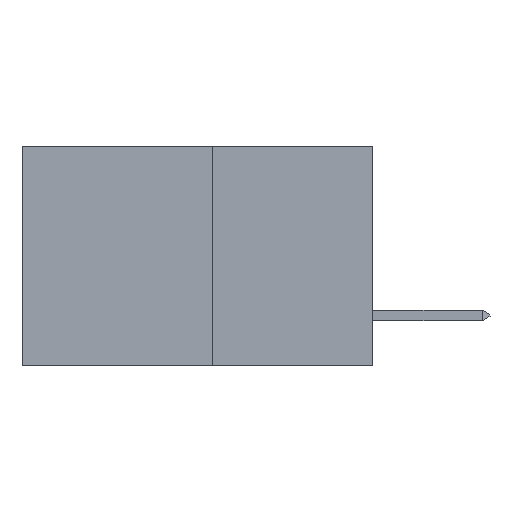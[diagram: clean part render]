
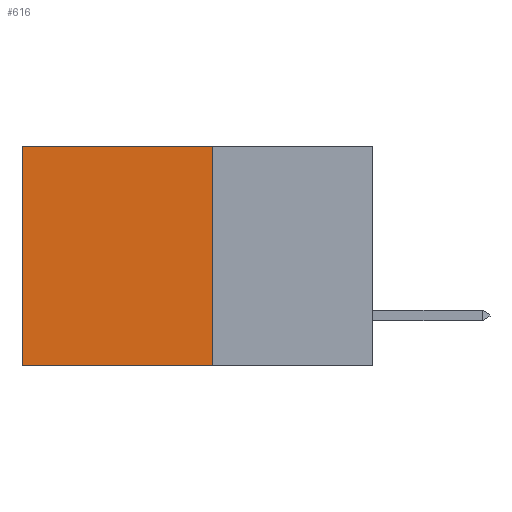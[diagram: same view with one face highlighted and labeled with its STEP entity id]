
A CAD part, left-side view. The second image highlights one B-rep face of the part: STEP entity #616.
In plain terms, the highlighted planar face has unit normal (-1, 0, 0).
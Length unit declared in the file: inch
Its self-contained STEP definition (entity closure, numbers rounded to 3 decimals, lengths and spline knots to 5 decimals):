
#457 = VERTEX_POINT ( 'NONE', #7300 ) ;
#496 = LINE ( 'NONE', #2315, #7386 ) ;
#616 = ADVANCED_FACE ( 'NONE', ( #7998 ), #9111, .F. ) ;
#890 = ORIENTED_EDGE ( 'NONE', *, *, #7282, .T. ) ;
#932 = DIRECTION ( 'NONE',  ( 0., 0., -1. ) ) ;
#1006 = LINE ( 'NONE', #1780, #9532 ) ;
#1780 = CARTESIAN_POINT ( 'NONE',  ( 0.277, 0.59, -0.37 ) ) ;
#1981 = DIRECTION ( 'NONE',  ( 0., 1., 0. ) ) ;
#2032 = AXIS2_PLACEMENT_3D ( 'NONE', #7136, #9435, #5856 ) ;
#2158 = EDGE_CURVE ( 'NONE', #7545, #8411, #9820, .T. ) ;
#2292 = DIRECTION ( 'NONE',  ( 0., 1., 0. ) ) ;
#2315 = CARTESIAN_POINT ( 'NONE',  ( 0.277, 0.27, 0. ) ) ;
#3061 = CARTESIAN_POINT ( 'NONE',  ( 0.277, 0.59, -0.37 ) ) ;
#3221 = ORIENTED_EDGE ( 'NONE', *, *, #2158, .F. ) ;
#3756 = VECTOR ( 'NONE', #9161, 39.37008 ) ;
#4755 = CARTESIAN_POINT ( 'NONE',  ( 0.277, 0.27, -0.37 ) ) ;
#4921 = EDGE_LOOP ( 'NONE', ( #8902, #3221, #7272, #890 ) ) ;
#5508 = VECTOR ( 'NONE', #2292, 39.37008 ) ;
#5856 = DIRECTION ( 'NONE',  ( 0., 0., -1. ) ) ;
#5879 = CARTESIAN_POINT ( 'NONE',  ( 0.277, 0.27, -0.37 ) ) ;
#7136 = CARTESIAN_POINT ( 'NONE',  ( 0.277, 0.27, -0.37 ) ) ;
#7272 = ORIENTED_EDGE ( 'NONE', *, *, #10523, .F. ) ;
#7282 = EDGE_CURVE ( 'NONE', #457, #8504, #496, .T. ) ;
#7300 = CARTESIAN_POINT ( 'NONE',  ( 0.277, 0.27, 0. ) ) ;
#7386 = VECTOR ( 'NONE', #1981, 39.37008 ) ;
#7394 = CARTESIAN_POINT ( 'NONE',  ( 0.277, 0.27, -0.37 ) ) ;
#7545 = VERTEX_POINT ( 'NONE', #4755 ) ;
#7998 = FACE_OUTER_BOUND ( 'NONE', #4921, .T. ) ;
#8143 = LINE ( 'NONE', #5879, #3756 ) ;
#8191 = CARTESIAN_POINT ( 'NONE',  ( 0.277, 0.59, 0. ) ) ;
#8411 = VERTEX_POINT ( 'NONE', #3061 ) ;
#8504 = VERTEX_POINT ( 'NONE', #8191 ) ;
#8902 = ORIENTED_EDGE ( 'NONE', *, *, #9360, .T. ) ;
#9111 = PLANE ( 'NONE',  #2032 ) ;
#9161 = DIRECTION ( 'NONE',  ( 0., 0., -1. ) ) ;
#9360 = EDGE_CURVE ( 'NONE', #8504, #8411, #1006, .T. ) ;
#9435 = DIRECTION ( 'NONE',  ( 1., 0., 0. ) ) ;
#9532 = VECTOR ( 'NONE', #932, 39.37008 ) ;
#9820 = LINE ( 'NONE', #7394, #5508 ) ;
#10523 = EDGE_CURVE ( 'NONE', #457, #7545, #8143, .T. ) ;
